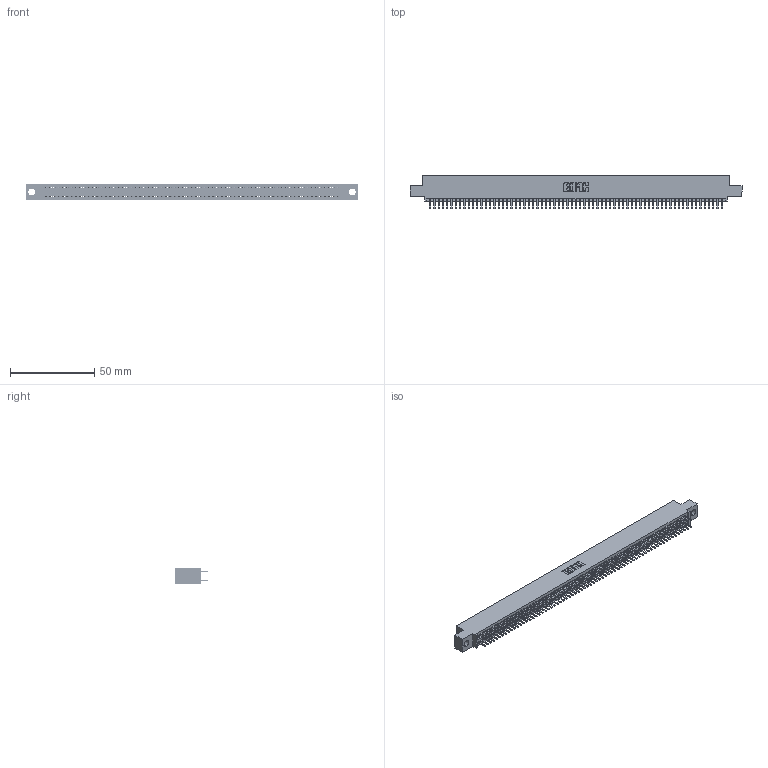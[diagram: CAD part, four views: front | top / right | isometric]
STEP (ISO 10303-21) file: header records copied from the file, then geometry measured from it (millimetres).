
FILE_DESCRIPTION (( 'STEP AP203' ), '1' );
FILE_NAME ('345-138-520-504.STEP', '2018-10-20T17:09:41', ( '' ), ( '' ), 'SwSTEP 2.0', 'SolidWorks 2016', '' );
FILE_SCHEMA (( 'CONFIG_CONTROL_DESIGN' ));
Length unit declared in the file: inch
Products named in the file (3): 345 Part_0.110 Offset - 0.156 Dia-TH; 345-292-001_345-293-120; 345-138-520-504
Assembly tree (139 placements, depth 2):
  345-138-520-504
    345 Part_0.110 Offset - 0.156 Dia-TH
    345-292-001_345-293-120  x138
Bounding box: 196.47 x 19.68 x 9.4 mm (x, y, z)
Volume: 19113.9 mm3; surface area: 28555.5 mm2
Topology: 139 solids, 139 shells, 7582 faces, 22019 edges, 14310 vertices
Faces by surface type: plane 4914, cylinder 2668
Entity records: 50753 total; most frequent: CARTESIAN_POINT 8496, ORIENTED_EDGE 8418, DIRECTION 7445, EDGE_CURVE 4209, LINE 3797, VECTOR 3797, VERTEX_POINT 2802, AXIS2_PLACEMENT_3D 1824
